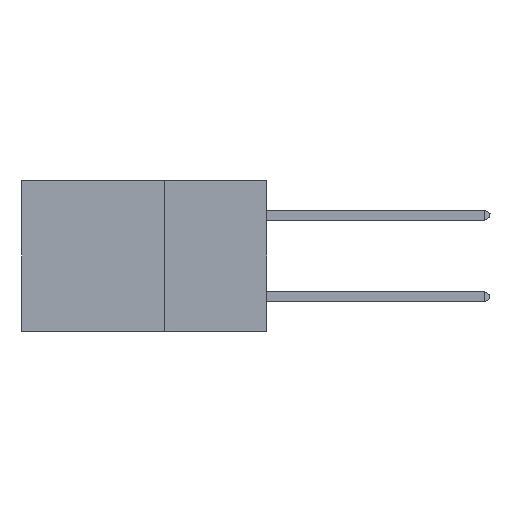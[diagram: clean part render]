
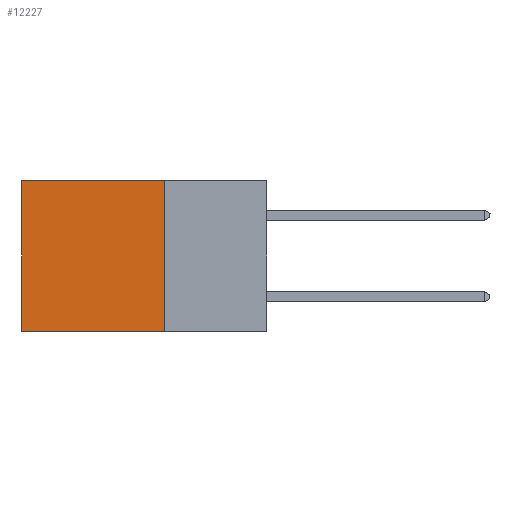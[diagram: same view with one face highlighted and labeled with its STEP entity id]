
A CAD part, left-side view. The second image highlights one B-rep face of the part: STEP entity #12227.
In plain terms, the highlighted planar face has unit normal (-1, 0, 0).
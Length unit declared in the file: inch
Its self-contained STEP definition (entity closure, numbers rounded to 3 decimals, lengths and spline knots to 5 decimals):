
#948 = ORIENTED_EDGE ( 'NONE', *, *, #4751, .F. ) ;
#1096 = VECTOR ( 'NONE', #4922, 39.37008 ) ;
#1319 = LINE ( 'NONE', #11681, #13258 ) ;
#2022 = CARTESIAN_POINT ( 'NONE',  ( 0.2875, 0.25, 0. ) ) ;
#2320 = DIRECTION ( 'NONE',  ( 0., 1., 0. ) ) ;
#2821 = VECTOR ( 'NONE', #18532, 39.37008 ) ;
#3458 = FACE_OUTER_BOUND ( 'NONE', #13362, .T. ) ;
#3767 = CARTESIAN_POINT ( 'NONE',  ( 0.2875, 0.25, -0.37 ) ) ;
#3914 = PLANE ( 'NONE',  #10297 ) ;
#4262 = EDGE_CURVE ( 'NONE', #9763, #14486, #9424, .T. ) ;
#4709 = VECTOR ( 'NONE', #13240, 39.37008 ) ;
#4751 = EDGE_CURVE ( 'NONE', #9763, #17431, #8905, .T. ) ;
#4922 = DIRECTION ( 'NONE',  ( 0., 1., 0. ) ) ;
#5478 = DIRECTION ( 'NONE',  ( 0., 0., -1. ) ) ;
#5704 = EDGE_CURVE ( 'NONE', #17431, #19713, #1319, .T. ) ;
#6275 = CARTESIAN_POINT ( 'NONE',  ( 0.2875, 0.6, -0.37 ) ) ;
#8905 = LINE ( 'NONE', #19095, #4709 ) ;
#9340 = ORIENTED_EDGE ( 'NONE', *, *, #4262, .T. ) ;
#9424 = LINE ( 'NONE', #16183, #1096 ) ;
#9763 = VERTEX_POINT ( 'NONE', #2022 ) ;
#10161 = CARTESIAN_POINT ( 'NONE',  ( 0.2875, 0.25, 0. ) ) ;
#10297 = AXIS2_PLACEMENT_3D ( 'NONE', #10161, #14796, #5478 ) ;
#10711 = ORIENTED_EDGE ( 'NONE', *, *, #16381, .T. ) ;
#10797 = CARTESIAN_POINT ( 'NONE',  ( 0.2875, 0.6, 0. ) ) ;
#10937 = CARTESIAN_POINT ( 'NONE',  ( 0.2875, 0.6, 0. ) ) ;
#11146 = LINE ( 'NONE', #10937, #2821 ) ;
#11681 = CARTESIAN_POINT ( 'NONE',  ( 0.2875, 0.25, -0.37 ) ) ;
#12227 = ADVANCED_FACE ( 'NONE', ( #3458 ), #3914, .F. ) ;
#13240 = DIRECTION ( 'NONE',  ( 0., 0., -1. ) ) ;
#13258 = VECTOR ( 'NONE', #2320, 39.37008 ) ;
#13362 = EDGE_LOOP ( 'NONE', ( #10711, #17329, #948, #9340 ) ) ;
#14486 = VERTEX_POINT ( 'NONE', #10797 ) ;
#14796 = DIRECTION ( 'NONE',  ( 1., 0., 0. ) ) ;
#16183 = CARTESIAN_POINT ( 'NONE',  ( 0.2875, 0.25, 0. ) ) ;
#16381 = EDGE_CURVE ( 'NONE', #14486, #19713, #11146, .T. ) ;
#17329 = ORIENTED_EDGE ( 'NONE', *, *, #5704, .F. ) ;
#17431 = VERTEX_POINT ( 'NONE', #3767 ) ;
#18532 = DIRECTION ( 'NONE',  ( 0., 0., -1. ) ) ;
#19095 = CARTESIAN_POINT ( 'NONE',  ( 0.2875, 0.25, 0. ) ) ;
#19713 = VERTEX_POINT ( 'NONE', #6275 ) ;
